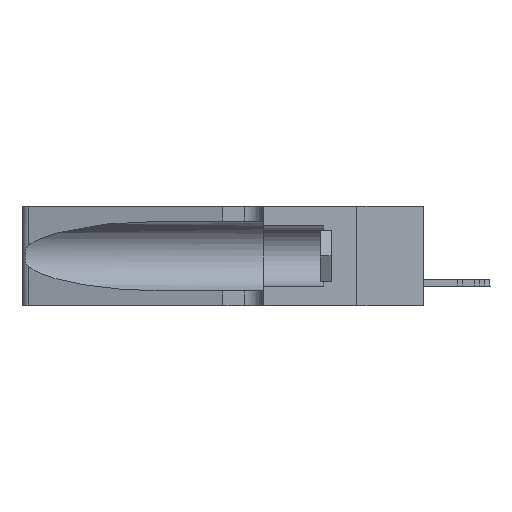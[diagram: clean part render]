
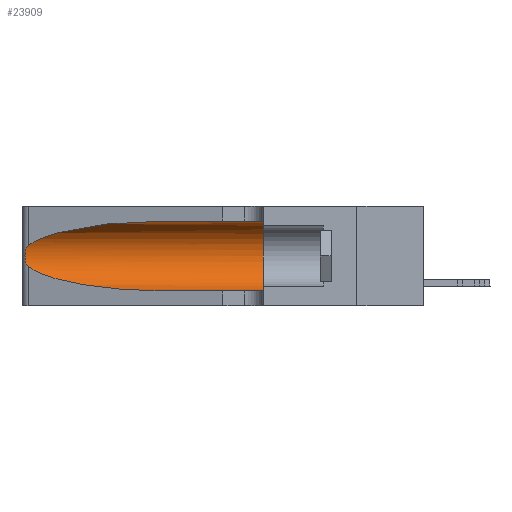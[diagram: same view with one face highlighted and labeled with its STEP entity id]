
A CAD part, left-side view. The second image highlights one B-rep face of the part: STEP entity #23909.
In plain terms, the highlighted cylindrical face has radius 3.308 mm (diameter 6.617 mm), a partial arc.
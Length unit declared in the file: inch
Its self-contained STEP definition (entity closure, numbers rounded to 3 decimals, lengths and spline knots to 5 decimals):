
#502 =( BOUNDED_CURVE ( )  B_SPLINE_CURVE ( 3, ( #35321, #15167, #39915, #29887 ),
 .UNSPECIFIED., .F., .T. ) 
 B_SPLINE_CURVE_WITH_KNOTS ( ( 4, 4 ),
 ( 3.44316, 4.71239 ),
 .UNSPECIFIED. ) 
 CURVE ( )  GEOMETRIC_REPRESENTATION_ITEM ( )  RATIONAL_B_SPLINE_CURVE ( ( 1., 0.87, 0.87, 1. ) ) 
 REPRESENTATION_ITEM ( '' )  );
#2029 = CARTESIAN_POINT ( 'NONE',  ( 0.25487, 1.22718, 0.22369 ) ) ;
#2902 = EDGE_CURVE ( 'NONE', #31852, #31407, #30306, .T. ) ;
#3334 = EDGE_CURVE ( 'NONE', #31852, #35283, #14304, .T. ) ;
#4142 = DIRECTION ( 'NONE',  ( 0., 0., -1. ) ) ;
#5654 = FACE_OUTER_BOUND ( 'NONE', #34164, .T. ) ;
#6622 = CARTESIAN_POINT ( 'NONE',  ( 0.25555, 1.22994, 0.2215 ) ) ;
#6958 = ORIENTED_EDGE ( 'NONE', *, *, #16393, .T. ) ;
#7457 = VECTOR ( 'NONE', #13274, 39.37008 ) ;
#8270 = ORIENTED_EDGE ( 'NONE', *, *, #26617, .F. ) ;
#8279 = CARTESIAN_POINT ( 'NONE',  ( 0.25789, 1.23486, 0.15765 ) ) ;
#8450 = CARTESIAN_POINT ( 'NONE',  ( 0.18966, 0.96281, 0.31525 ) ) ;
#9311 = CYLINDRICAL_SURFACE ( 'NONE', #10278, 0.13025 ) ;
#10278 = AXIS2_PLACEMENT_3D ( 'NONE', #33054, #35971, #4142 ) ;
#10979 = CARTESIAN_POINT ( 'NONE',  ( 0.25854, 1.2359, 0.20912 ) ) ;
#12605 = EDGE_CURVE ( 'NONE', #30691, #18162, #43117, .T. ) ;
#13274 = DIRECTION ( 'NONE',  ( 0., -1., 0. ) ) ;
#13534 = CARTESIAN_POINT ( 'NONE',  ( 0.25487, 1.22718, 0.22369 ) ) ;
#13781 = CARTESIAN_POINT ( 'NONE',  ( 0.25487, 1.22718, 0.22369 ) ) ;
#14304 = LINE ( 'NONE', #26731, #7457 ) ;
#15167 = CARTESIAN_POINT ( 'NONE',  ( 0.2373, 1.15595, 0.08982 ) ) ;
#15380 = CARTESIAN_POINT ( 'NONE',  ( 0.2373, 1.15595, 0.28018 ) ) ;
#16178 = B_SPLINE_CURVE_WITH_KNOTS ( 'NONE', 3,
 ( #13781, #6622, #26964, #24390, #10979, #34701, #18521, #36098, #37701, #28452, #8279, #17702, #41281, #18616 ),
 .UNSPECIFIED., .F., .F.,
 ( 4, 2, 2, 2, 2, 2, 4 ),
 ( 0., 0.00027, 0.00053, 0.00107, 0.0016, 0.00187, 0.00214 ),
 .UNSPECIFIED. ) ;
#16393 = EDGE_CURVE ( 'NONE', #31407, #26425, #16178, .T. ) ;
#16842 = EDGE_CURVE ( 'NONE', #26425, #30691, #502, .T. ) ;
#17702 = CARTESIAN_POINT ( 'NONE',  ( 0.25639, 1.23186, 0.15144 ) ) ;
#18127 = CIRCLE ( 'NONE', #18679, 0.13025 ) ;
#18162 = VERTEX_POINT ( 'NONE', #42548 ) ;
#18521 = CARTESIAN_POINT ( 'NONE',  ( 0.26075, 1.23896, 0.19203 ) ) ;
#18616 = CARTESIAN_POINT ( 'NONE',  ( 0.25487, 1.22718, 0.14631 ) ) ;
#18679 = AXIS2_PLACEMENT_3D ( 'NONE', #34271, #40724, #40589 ) ;
#18946 = ORIENTED_EDGE ( 'NONE', *, *, #2902, .T. ) ;
#19155 = CARTESIAN_POINT ( 'NONE',  ( 0.1305, 0.72297, 0.31525 ) ) ;
#21081 = CARTESIAN_POINT ( 'NONE',  ( 0.25487, 1.22718, 0.14631 ) ) ;
#22994 = CARTESIAN_POINT ( 'NONE',  ( 0.1305, 1.61858, 0.05475 ) ) ;
#23419 = DIRECTION ( 'NONE',  ( 0., -1., 0. ) ) ;
#23909 = ADVANCED_FACE ( 'NONE', ( #5654 ), #9311, .F. ) ;
#24390 = CARTESIAN_POINT ( 'NONE',  ( 0.25787, 1.23484, 0.2124 ) ) ;
#26425 = VERTEX_POINT ( 'NONE', #21081 ) ;
#26617 = EDGE_CURVE ( 'NONE', #35283, #18162, #18127, .T. ) ;
#26731 = CARTESIAN_POINT ( 'NONE',  ( 0.1305, 1.61858, 0.31525 ) ) ;
#26964 = CARTESIAN_POINT ( 'NONE',  ( 0.25639, 1.23184, 0.21858 ) ) ;
#28452 = CARTESIAN_POINT ( 'NONE',  ( 0.25856, 1.23593, 0.16098 ) ) ;
#29688 = CARTESIAN_POINT ( 'NONE',  ( 0.1305, 0.72297, 0.05475 ) ) ;
#29887 = CARTESIAN_POINT ( 'NONE',  ( 0.1305, 0.72297, 0.05475 ) ) ;
#30306 =( BOUNDED_CURVE ( )  B_SPLINE_CURVE ( 3, ( #19155, #8450, #15380, #2029 ),
 .UNSPECIFIED., .F., .F. ) 
 B_SPLINE_CURVE_WITH_KNOTS ( ( 4, 4 ),
 ( 1.5708, 2.84003 ),
 .UNSPECIFIED. ) 
 CURVE ( )  GEOMETRIC_REPRESENTATION_ITEM ( )  RATIONAL_B_SPLINE_CURVE ( ( 1., 0.87, 0.87, 1. ) ) 
 REPRESENTATION_ITEM ( '' )  );
#30691 = VERTEX_POINT ( 'NONE', #29688 ) ;
#31407 = VERTEX_POINT ( 'NONE', #13534 ) ;
#31852 = VERTEX_POINT ( 'NONE', #39050 ) ;
#33054 = CARTESIAN_POINT ( 'NONE',  ( 0.1305, 1.61858, 0.185 ) ) ;
#34164 = EDGE_LOOP ( 'NONE', ( #18946, #6958, #39958, #41684, #8270, #41748 ) ) ;
#34271 = CARTESIAN_POINT ( 'NONE',  ( 0.1305, 0.35, 0.185 ) ) ;
#34701 = CARTESIAN_POINT ( 'NONE',  ( 0.26018, 1.23835, 0.19895 ) ) ;
#35283 = VERTEX_POINT ( 'NONE', #41432 ) ;
#35321 = CARTESIAN_POINT ( 'NONE',  ( 0.25487, 1.22718, 0.14631 ) ) ;
#35971 = DIRECTION ( 'NONE',  ( 0., -1., 0. ) ) ;
#36098 = CARTESIAN_POINT ( 'NONE',  ( 0.26075, 1.23896, 0.178 ) ) ;
#37701 = CARTESIAN_POINT ( 'NONE',  ( 0.26017, 1.23833, 0.17102 ) ) ;
#39050 = CARTESIAN_POINT ( 'NONE',  ( 0.1305, 0.72297, 0.31525 ) ) ;
#39915 = CARTESIAN_POINT ( 'NONE',  ( 0.18966, 0.96281, 0.05475 ) ) ;
#39958 = ORIENTED_EDGE ( 'NONE', *, *, #16842, .T. ) ;
#40437 = VECTOR ( 'NONE', #23419, 39.37008 ) ;
#40589 = DIRECTION ( 'NONE',  ( 0., 0., 1. ) ) ;
#40724 = DIRECTION ( 'NONE',  ( 0., 1., 0. ) ) ;
#41281 = CARTESIAN_POINT ( 'NONE',  ( 0.25555, 1.22993, 0.14849 ) ) ;
#41432 = CARTESIAN_POINT ( 'NONE',  ( 0.1305, 0.35, 0.31525 ) ) ;
#41684 = ORIENTED_EDGE ( 'NONE', *, *, #12605, .T. ) ;
#41748 = ORIENTED_EDGE ( 'NONE', *, *, #3334, .F. ) ;
#42548 = CARTESIAN_POINT ( 'NONE',  ( 0.1305, 0.35, 0.05475 ) ) ;
#43117 = LINE ( 'NONE', #22994, #40437 ) ;
